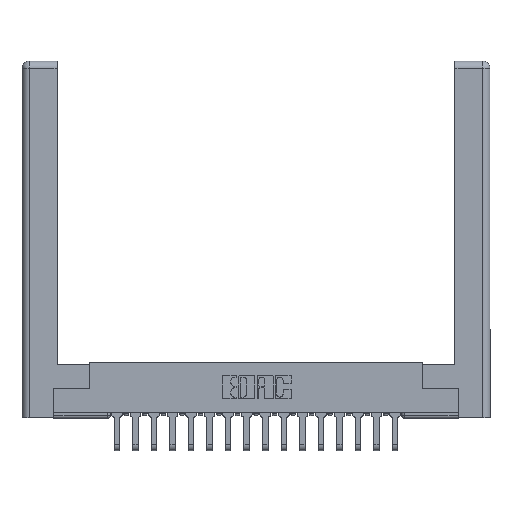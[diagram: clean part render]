
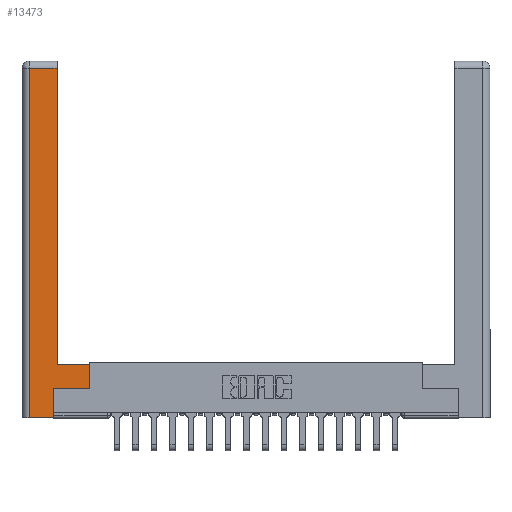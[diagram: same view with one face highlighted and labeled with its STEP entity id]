
A CAD part, top view. The second image highlights one B-rep face of the part: STEP entity #13473.
In plain terms, the highlighted planar face has unit normal (0, 0, 1).
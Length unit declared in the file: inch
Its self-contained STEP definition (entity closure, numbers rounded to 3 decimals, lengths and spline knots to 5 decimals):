
#75 = ORIENTED_EDGE ( 'NONE', *, *, #18896, .T. ) ;
#264 = VECTOR ( 'NONE', #17105, 39.37008 ) ;
#672 = DIRECTION ( 'NONE',  ( -1., 0., 0. ) ) ;
#739 = CARTESIAN_POINT ( 'NONE',  ( 0., 0., 0. ) ) ;
#875 = DIRECTION ( 'NONE',  ( 0., 0., -1. ) ) ;
#988 = VERTEX_POINT ( 'NONE', #1709 ) ;
#1314 = ORIENTED_EDGE ( 'NONE', *, *, #4531, .T. ) ;
#1709 = CARTESIAN_POINT ( 'NONE',  ( 0.265, 0., 0. ) ) ;
#1871 = LINE ( 'NONE', #9831, #3045 ) ;
#1885 = DIRECTION ( 'NONE',  ( -1., 0., 0. ) ) ;
#2135 = DIRECTION ( 'NONE',  ( 1., 0., 0. ) ) ;
#2226 = VERTEX_POINT ( 'NONE', #18868 ) ;
#2342 = DIRECTION ( 'NONE',  ( 1., 0., 0. ) ) ;
#2963 = CARTESIAN_POINT ( 'NONE',  ( 0.0615, 0., 0. ) ) ;
#3045 = VECTOR ( 'NONE', #2342, 39.37008 ) ;
#3493 = VECTOR ( 'NONE', #9349, 39.37008 ) ;
#3777 = FACE_OUTER_BOUND ( 'NONE', #13150, .T. ) ;
#4306 = VERTEX_POINT ( 'NONE', #17941 ) ;
#4531 = EDGE_CURVE ( 'NONE', #6471, #7456, #14103, .T. ) ;
#4561 = LINE ( 'NONE', #17295, #264 ) ;
#4895 = VERTEX_POINT ( 'NONE', #2963 ) ;
#5117 = VECTOR ( 'NONE', #16943, 39.37008 ) ;
#5666 = ORIENTED_EDGE ( 'NONE', *, *, #19440, .T. ) ;
#5692 = LINE ( 'NONE', #14067, #17570 ) ;
#6195 = ORIENTED_EDGE ( 'NONE', *, *, #7067, .T. ) ;
#6342 = LINE ( 'NONE', #12536, #3493 ) ;
#6471 = VERTEX_POINT ( 'NONE', #13317 ) ;
#7042 = ORIENTED_EDGE ( 'NONE', *, *, #7663, .T. ) ;
#7044 = ORIENTED_EDGE ( 'NONE', *, *, #16236, .T. ) ;
#7067 = EDGE_CURVE ( 'NONE', #10424, #4306, #12131, .T. ) ;
#7144 = VECTOR ( 'NONE', #1885, 39.37008 ) ;
#7456 = VERTEX_POINT ( 'NONE', #9096 ) ;
#7663 = EDGE_CURVE ( 'NONE', #2226, #10424, #5692, .T. ) ;
#7835 = LINE ( 'NONE', #18348, #7144 ) ;
#8201 = LINE ( 'NONE', #12237, #5117 ) ;
#9096 = CARTESIAN_POINT ( 'NONE',  ( 0.0615, 2.94, 0. ) ) ;
#9294 = DIRECTION ( 'NONE',  ( -1., 0., 0. ) ) ;
#9334 = EDGE_CURVE ( 'NONE', #988, #2226, #8201, .T. ) ;
#9349 = DIRECTION ( 'NONE',  ( 0., -1., 0. ) ) ;
#9831 = CARTESIAN_POINT ( 'NONE',  ( 0.265, 0., 0. ) ) ;
#10424 = VERTEX_POINT ( 'NONE', #18278 ) ;
#10593 = AXIS2_PLACEMENT_3D ( 'NONE', #739, #875, #672 ) ;
#10867 = CARTESIAN_POINT ( 'NONE',  ( 0.295, 0.45, 0. ) ) ;
#11348 = ORIENTED_EDGE ( 'NONE', *, *, #9334, .T. ) ;
#11446 = ORIENTED_EDGE ( 'NONE', *, *, #15804, .T. ) ;
#12131 = LINE ( 'NONE', #12715, #17353 ) ;
#12237 = CARTESIAN_POINT ( 'NONE',  ( 0.265, 0.245, 0. ) ) ;
#12536 = CARTESIAN_POINT ( 'NONE',  ( 0.0615, 0., 0. ) ) ;
#12553 = CARTESIAN_POINT ( 'NONE',  ( 0.0615, 2.94, 0. ) ) ;
#12715 = CARTESIAN_POINT ( 'NONE',  ( 0.565, 0.45, 0. ) ) ;
#13150 = EDGE_LOOP ( 'NONE', ( #75, #1314, #7044, #11446, #11348, #7042, #6195, #5666 ) ) ;
#13317 = CARTESIAN_POINT ( 'NONE',  ( 0.295, 2.94, 0. ) ) ;
#13473 = ADVANCED_FACE ( 'NONE', ( #3777 ), #16169, .F. ) ;
#14067 = CARTESIAN_POINT ( 'NONE',  ( 0.565, 0.245, 0. ) ) ;
#14103 = LINE ( 'NONE', #12553, #17682 ) ;
#14404 = VERTEX_POINT ( 'NONE', #10867 ) ;
#15804 = EDGE_CURVE ( 'NONE', #4895, #988, #1871, .T. ) ;
#16169 = PLANE ( 'NONE',  #10593 ) ;
#16236 = EDGE_CURVE ( 'NONE', #7456, #4895, #6342, .T. ) ;
#16943 = DIRECTION ( 'NONE',  ( 0., 1., 0. ) ) ;
#17105 = DIRECTION ( 'NONE',  ( 0., 1., 0. ) ) ;
#17163 = DIRECTION ( 'NONE',  ( 0., 1., 0. ) ) ;
#17295 = CARTESIAN_POINT ( 'NONE',  ( 0.295, 3., 0. ) ) ;
#17353 = VECTOR ( 'NONE', #17163, 39.37008 ) ;
#17570 = VECTOR ( 'NONE', #2135, 39.37008 ) ;
#17682 = VECTOR ( 'NONE', #9294, 39.37008 ) ;
#17941 = CARTESIAN_POINT ( 'NONE',  ( 0.565, 0.45, 0. ) ) ;
#18278 = CARTESIAN_POINT ( 'NONE',  ( 0.565, 0.245, 0. ) ) ;
#18348 = CARTESIAN_POINT ( 'NONE',  ( 0.295, 0.45, 0. ) ) ;
#18868 = CARTESIAN_POINT ( 'NONE',  ( 0.265, 0.245, 0. ) ) ;
#18896 = EDGE_CURVE ( 'NONE', #14404, #6471, #4561, .T. ) ;
#19440 = EDGE_CURVE ( 'NONE', #4306, #14404, #7835, .T. ) ;
